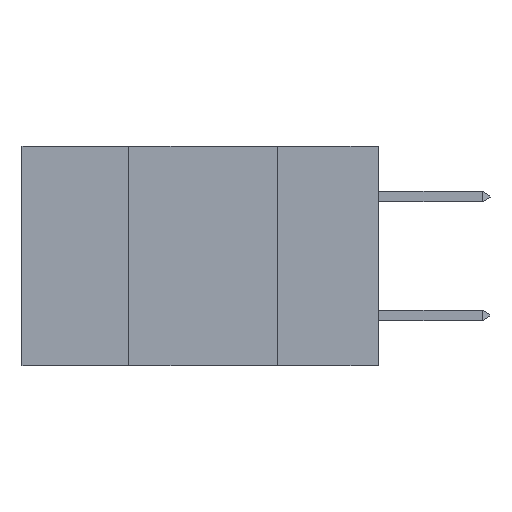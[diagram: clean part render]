
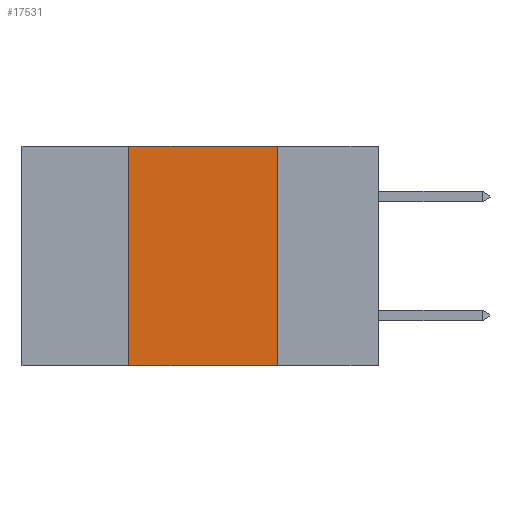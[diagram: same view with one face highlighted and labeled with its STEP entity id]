
A CAD part, left-side view. The second image highlights one B-rep face of the part: STEP entity #17531.
In plain terms, the highlighted planar face has unit normal (-1, 0, 0).
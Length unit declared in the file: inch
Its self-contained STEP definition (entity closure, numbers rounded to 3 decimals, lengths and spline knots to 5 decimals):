
#1521 = ORIENTED_EDGE ( 'NONE', *, *, #4449, .T. ) ;
#1673 = DIRECTION ( 'NONE',  ( 1., 0., 0. ) ) ;
#1920 = CARTESIAN_POINT ( 'NONE',  ( 0., 0.42, -0.37 ) ) ;
#3462 = VECTOR ( 'NONE', #19115, 39.37008 ) ;
#3847 = DIRECTION ( 'NONE',  ( 0., -1., 0. ) ) ;
#4158 = CARTESIAN_POINT ( 'NONE',  ( 0., 0.17, -0.37 ) ) ;
#4395 = ORIENTED_EDGE ( 'NONE', *, *, #8643, .F. ) ;
#4449 = EDGE_CURVE ( 'NONE', #23563, #21832, #9657, .T. ) ;
#5437 = EDGE_LOOP ( 'NONE', ( #15082, #14578, #4395, #1521 ) ) ;
#6239 = DIRECTION ( 'NONE',  ( 0., 0., -1. ) ) ;
#7245 = CARTESIAN_POINT ( 'NONE',  ( 0., 0.17, -0.37 ) ) ;
#8299 = LINE ( 'NONE', #4158, #18636 ) ;
#8643 = EDGE_CURVE ( 'NONE', #23563, #20477, #16384, .T. ) ;
#9657 = LINE ( 'NONE', #21642, #3462 ) ;
#11168 = AXIS2_PLACEMENT_3D ( 'NONE', #12021, #1673, #16171 ) ;
#12021 = CARTESIAN_POINT ( 'NONE',  ( 0., 0.6, 0. ) ) ;
#12798 = EDGE_CURVE ( 'NONE', #20477, #16558, #12963, .T. ) ;
#12865 = CARTESIAN_POINT ( 'NONE',  ( 0., 0.42, -0.37 ) ) ;
#12963 = LINE ( 'NONE', #14174, #17797 ) ;
#14174 = CARTESIAN_POINT ( 'NONE',  ( 0., 0.6, 0. ) ) ;
#14578 = ORIENTED_EDGE ( 'NONE', *, *, #12798, .F. ) ;
#15082 = ORIENTED_EDGE ( 'NONE', *, *, #16932, .F. ) ;
#16047 = FACE_OUTER_BOUND ( 'NONE', #5437, .T. ) ;
#16171 = DIRECTION ( 'NONE',  ( 0., 0., -1. ) ) ;
#16384 = LINE ( 'NONE', #1920, #26038 ) ;
#16558 = VERTEX_POINT ( 'NONE', #25477 ) ;
#16932 = EDGE_CURVE ( 'NONE', #16558, #21832, #8299, .T. ) ;
#17531 = ADVANCED_FACE ( 'NONE', ( #16047 ), #26408, .F. ) ;
#17797 = VECTOR ( 'NONE', #3847, 39.37008 ) ;
#18636 = VECTOR ( 'NONE', #6239, 39.37008 ) ;
#19115 = DIRECTION ( 'NONE',  ( 0., -1., 0. ) ) ;
#20477 = VERTEX_POINT ( 'NONE', #26453 ) ;
#21642 = CARTESIAN_POINT ( 'NONE',  ( 0., 0.6, -0.37 ) ) ;
#21832 = VERTEX_POINT ( 'NONE', #7245 ) ;
#23563 = VERTEX_POINT ( 'NONE', #12865 ) ;
#24601 = DIRECTION ( 'NONE',  ( 0., 0., 1. ) ) ;
#25477 = CARTESIAN_POINT ( 'NONE',  ( 0., 0.17, 0. ) ) ;
#26038 = VECTOR ( 'NONE', #24601, 39.37008 ) ;
#26408 = PLANE ( 'NONE',  #11168 ) ;
#26453 = CARTESIAN_POINT ( 'NONE',  ( 0., 0.42, 0. ) ) ;
